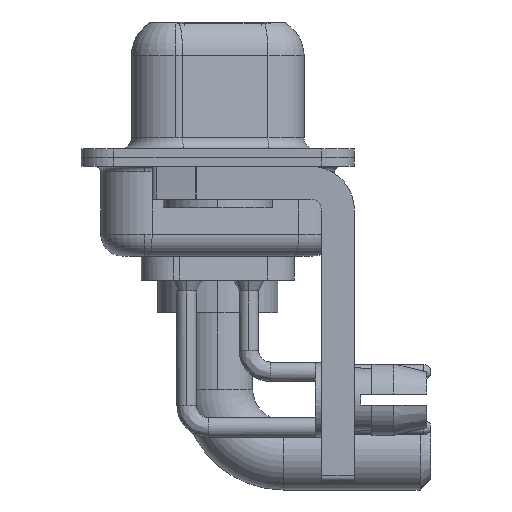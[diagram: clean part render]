
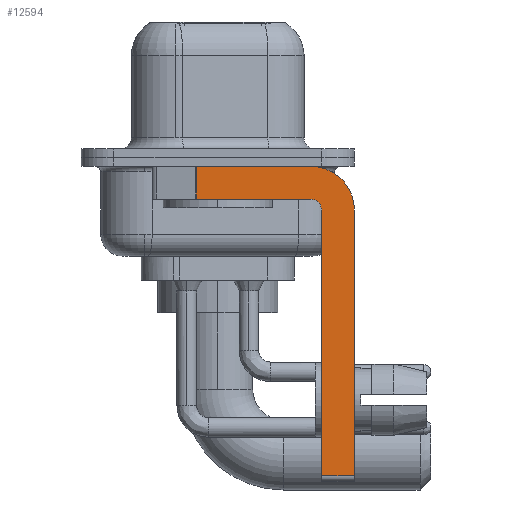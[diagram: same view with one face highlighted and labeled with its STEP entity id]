
A CAD part, left-side view. The second image highlights one B-rep face of the part: STEP entity #12594.
In plain terms, the highlighted planar face has unit normal (-1, 0, 0).
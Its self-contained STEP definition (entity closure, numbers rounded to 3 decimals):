
#42 = CARTESIAN_POINT ( 'NONE',  ( -2.9, -6.25, -2.4 ) ) ;
#114 = CARTESIAN_POINT ( 'NONE',  ( -2.9, -4.75, -2.4 ) ) ;
#118 = CARTESIAN_POINT ( 'NONE',  ( -2.9, -4.25, -2.4 ) ) ;
#242 = ORIENTED_EDGE ( 'NONE', *, *, #8883, .F. ) ;
#335 = DIRECTION ( 'NONE',  ( 0., 0., -1. ) ) ;
#615 = PLANE ( 'NONE',  #20931 ) ;
#904 = EDGE_CURVE ( 'NONE', #4010, #14434, #14496, .T. ) ;
#1119 = LINE ( 'NONE', #7637, #14722 ) ;
#1197 = ORIENTED_EDGE ( 'NONE', *, *, #904, .T. ) ;
#1509 = CARTESIAN_POINT ( 'NONE',  ( -2.9, -4.25, -2.4 ) ) ;
#1831 = DIRECTION ( 'NONE',  ( 0., 0., 1. ) ) ;
#3186 = EDGE_LOOP ( 'NONE', ( #11107, #1197, #20862, #242, #11479, #11437, #19868, #10927 ) ) ;
#3837 = FACE_OUTER_BOUND ( 'NONE', #3186, .T. ) ;
#4010 = VERTEX_POINT ( 'NONE', #11532 ) ;
#4633 = EDGE_CURVE ( 'NONE', #4010, #7745, #10249, .T. ) ;
#4684 = CARTESIAN_POINT ( 'NONE',  ( -2.9, 0.978, -1.9 ) ) ;
#5258 = DIRECTION ( 'NONE',  ( 1., 0., 0. ) ) ;
#5731 = DIRECTION ( 'NONE',  ( 1., 0., 0. ) ) ;
#6223 = CIRCLE ( 'NONE', #16443, 2. ) ;
#6234 = DIRECTION ( 'NONE',  ( 0., 1., 0. ) ) ;
#6755 = CARTESIAN_POINT ( 'NONE',  ( -2.9, -4.25, -14.55 ) ) ;
#7249 = CARTESIAN_POINT ( 'NONE',  ( -2.9, 3., -0.4 ) ) ;
#7270 = CIRCLE ( 'NONE', #7609, 0.5 ) ;
#7330 = EDGE_CURVE ( 'NONE', #18776, #8922, #15359, .T. ) ;
#7513 = VECTOR ( 'NONE', #20912, 1000. ) ;
#7609 = AXIS2_PLACEMENT_3D ( 'NONE', #1509, #19526, #1831 ) ;
#7637 = CARTESIAN_POINT ( 'NONE',  ( -2.9, -4.25, -1.9 ) ) ;
#7745 = VERTEX_POINT ( 'NONE', #16929 ) ;
#8725 = VECTOR ( 'NONE', #16031, 1000. ) ;
#8883 = EDGE_CURVE ( 'NONE', #8922, #15455, #7270, .T. ) ;
#8922 = VERTEX_POINT ( 'NONE', #114 ) ;
#9643 = EDGE_CURVE ( 'NONE', #15455, #14434, #1119, .T. ) ;
#9732 = VERTEX_POINT ( 'NONE', #19659 ) ;
#9823 = VECTOR ( 'NONE', #16565, 1000. ) ;
#10089 = EDGE_CURVE ( 'NONE', #7745, #9732, #6223, .T. ) ;
#10249 = LINE ( 'NONE', #7249, #14581 ) ;
#10354 = DIRECTION ( 'NONE',  ( 0., -1., 0. ) ) ;
#10462 = CARTESIAN_POINT ( 'NONE',  ( -2.9, -4.75, -14.8 ) ) ;
#10927 = ORIENTED_EDGE ( 'NONE', *, *, #10089, .F. ) ;
#11107 = ORIENTED_EDGE ( 'NONE', *, *, #4633, .F. ) ;
#11437 = ORIENTED_EDGE ( 'NONE', *, *, #19839, .T. ) ;
#11479 = ORIENTED_EDGE ( 'NONE', *, *, #7330, .F. ) ;
#11532 = CARTESIAN_POINT ( 'NONE',  ( -2.9, 0.978, -0.4 ) ) ;
#11547 = LINE ( 'NONE', #6755, #9823 ) ;
#11626 = CARTESIAN_POINT ( 'NONE',  ( -2.9, 0.978, -1.9 ) ) ;
#12303 = VECTOR ( 'NONE', #20262, 1000. ) ;
#12594 = ADVANCED_FACE ( 'NONE', ( #3837 ), #615, .F. ) ;
#14117 = VERTEX_POINT ( 'NONE', #18010 ) ;
#14434 = VERTEX_POINT ( 'NONE', #4684 ) ;
#14496 = LINE ( 'NONE', #11626, #7513 ) ;
#14581 = VECTOR ( 'NONE', #10354, 1000. ) ;
#14722 = VECTOR ( 'NONE', #6234, 1000. ) ;
#15326 = CARTESIAN_POINT ( 'NONE',  ( -2.9, -4.25, -2.4 ) ) ;
#15359 = LINE ( 'NONE', #10462, #12303 ) ;
#15455 = VERTEX_POINT ( 'NONE', #16047 ) ;
#16031 = DIRECTION ( 'NONE',  ( 0., 0., -1. ) ) ;
#16047 = CARTESIAN_POINT ( 'NONE',  ( -2.9, -4.25, -1.9 ) ) ;
#16132 = LINE ( 'NONE', #42, #8725 ) ;
#16443 = AXIS2_PLACEMENT_3D ( 'NONE', #118, #5258, #335 ) ;
#16565 = DIRECTION ( 'NONE',  ( 0., -1., 0. ) ) ;
#16574 = CARTESIAN_POINT ( 'NONE',  ( -2.9, -4.75, -14.55 ) ) ;
#16929 = CARTESIAN_POINT ( 'NONE',  ( -2.9, -4.25, -0.4 ) ) ;
#17186 = EDGE_CURVE ( 'NONE', #9732, #14117, #16132, .T. ) ;
#18010 = CARTESIAN_POINT ( 'NONE',  ( -2.9, -6.25, -14.55 ) ) ;
#18412 = DIRECTION ( 'NONE',  ( 0., 0., -1. ) ) ;
#18776 = VERTEX_POINT ( 'NONE', #16574 ) ;
#19526 = DIRECTION ( 'NONE',  ( -1., 0., 0. ) ) ;
#19659 = CARTESIAN_POINT ( 'NONE',  ( -2.9, -6.25, -2.4 ) ) ;
#19839 = EDGE_CURVE ( 'NONE', #18776, #14117, #11547, .T. ) ;
#19868 = ORIENTED_EDGE ( 'NONE', *, *, #17186, .F. ) ;
#20262 = DIRECTION ( 'NONE',  ( 0., 0., 1. ) ) ;
#20862 = ORIENTED_EDGE ( 'NONE', *, *, #9643, .F. ) ;
#20912 = DIRECTION ( 'NONE',  ( 0., 0., -1. ) ) ;
#20931 = AXIS2_PLACEMENT_3D ( 'NONE', #15326, #5731, #18412 ) ;
